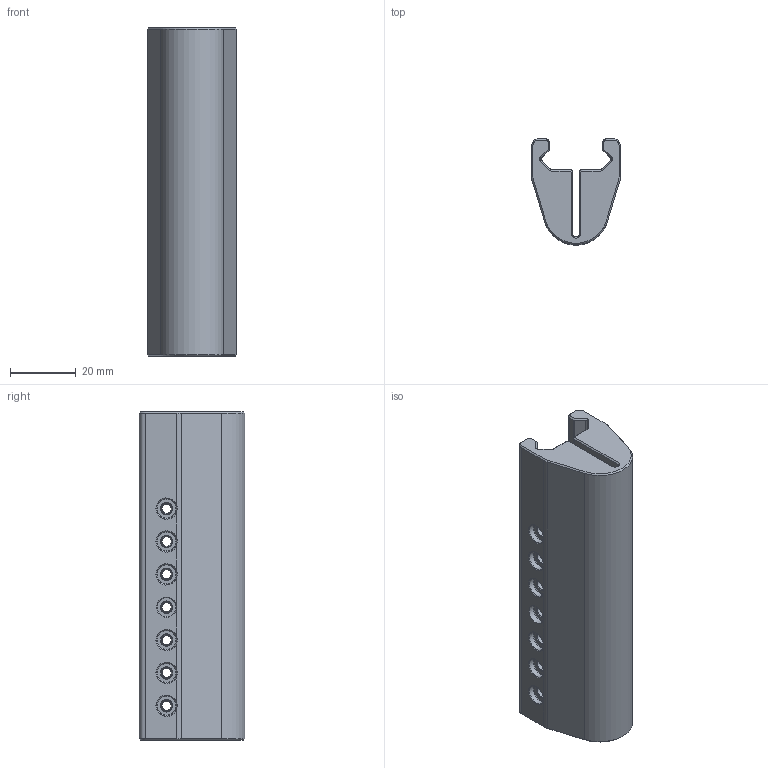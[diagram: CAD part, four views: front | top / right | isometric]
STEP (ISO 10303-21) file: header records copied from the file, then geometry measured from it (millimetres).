
FILE_DESCRIPTION(/* description */ (''),/* implementation_level */ '2;1');
FILE_NAME(/* name */ 'bag_rider.step',/* time_stamp */ '2023-12-22T00:03:46+13:00',/* author */ (''),/* organization */ (''),/* preprocessor_version */ 'ST-DEVELOPER v20',/* originating_system */ 'Autodesk Translation Framework v12.14.0.127',/* authorisation */ '');
FILE_SCHEMA (('AUTOMOTIVE_DESIGN { 1 0 10303 214 3 1 1 }'));
Length unit declared in the file: millimetre
Products named in the file (1): at-x bag rider
Bounding box: 27 x 32.16 x 100 mm (x, y, z)
Volume: 50839.1 mm3; surface area: 17763.3 mm2
Topology: 1 solids, 1 shells, 216 faces, 562 edges, 335 vertices
Faces by surface type: cylinder 72, plane 71, cone 59, torus 14
Full cylindrical faces by diameter (mm): 2.8 x7, 3.4 x7, 6.1 x7
Entity records: 7043 total; most frequent: CARTESIAN_POINT 1732, ORIENTED_EDGE 1124, DIRECTION 1108, EDGE_CURVE 562, AXIS2_PLACEMENT_3D 405, VERTEX_POINT 335, LINE 298, VECTOR 298
